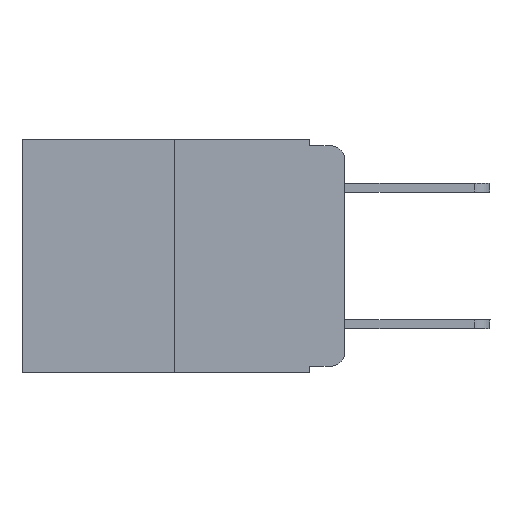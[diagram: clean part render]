
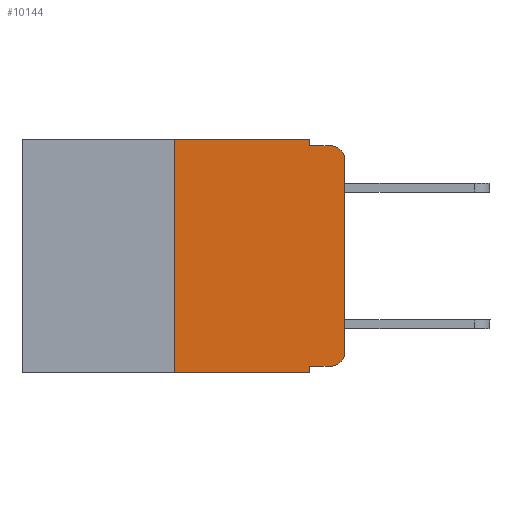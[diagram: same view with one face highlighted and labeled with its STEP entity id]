
A CAD part, left-side view. The second image highlights one B-rep face of the part: STEP entity #10144.
In plain terms, the highlighted planar face has unit normal (-1, 0, 0).
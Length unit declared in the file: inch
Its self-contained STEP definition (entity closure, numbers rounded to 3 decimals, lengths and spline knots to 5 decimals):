
#7 = VERTEX_POINT ( 'NONE', #2720 ) ;
#46 = VERTEX_POINT ( 'NONE', #10222 ) ;
#53 = CARTESIAN_POINT ( 'NONE',  ( 0., 0.473, 0. ) ) ;
#612 = EDGE_CURVE ( 'NONE', #9801, #11192, #1618, .T. ) ;
#665 = FACE_OUTER_BOUND ( 'NONE', #2804, .T. ) ;
#757 = VECTOR ( 'NONE', #13112, 39.37008 ) ;
#1038 = LINE ( 'NONE', #6420, #1865 ) ;
#1233 = AXIS2_PLACEMENT_3D ( 'NONE', #4231, #5417, #5269 ) ;
#1427 = ORIENTED_EDGE ( 'NONE', *, *, #6035, .F. ) ;
#1511 = DIRECTION ( 'NONE',  ( 0., 0., 1. ) ) ;
#1618 = LINE ( 'NONE', #6082, #13371 ) ;
#1855 = CIRCLE ( 'NONE', #6973, 0.02 ) ;
#1865 = VECTOR ( 'NONE', #6332, 39.37008 ) ;
#1982 = CARTESIAN_POINT ( 'NONE',  ( 0., 0.473, 0. ) ) ;
#2523 = ORIENTED_EDGE ( 'NONE', *, *, #2851, .F. ) ;
#2578 = EDGE_CURVE ( 'NONE', #7189, #3994, #7212, .T. ) ;
#2700 = LINE ( 'NONE', #53, #11826 ) ;
#2720 = CARTESIAN_POINT ( 'NONE',  ( 0., 0., -0.313 ) ) ;
#2748 = DIRECTION ( 'NONE',  ( -1., 0., 0. ) ) ;
#2804 = EDGE_LOOP ( 'NONE', ( #5106, #3566, #2523, #9896, #1427, #4032, #12704, #13090, #8368, #5685 ) ) ;
#2851 = EDGE_CURVE ( 'NONE', #3994, #3836, #1038, .T. ) ;
#2891 = DIRECTION ( 'NONE',  ( 0., -1., 0. ) ) ;
#3566 = ORIENTED_EDGE ( 'NONE', *, *, #7395, .T. ) ;
#3836 = VERTEX_POINT ( 'NONE', #6130 ) ;
#3950 = CARTESIAN_POINT ( 'NONE',  ( 0., 0., -0.03 ) ) ;
#3974 = LINE ( 'NONE', #6555, #12480 ) ;
#3994 = VERTEX_POINT ( 'NONE', #9309 ) ;
#4032 = ORIENTED_EDGE ( 'NONE', *, *, #4300, .F. ) ;
#4059 = VERTEX_POINT ( 'NONE', #10612 ) ;
#4231 = CARTESIAN_POINT ( 'NONE',  ( 0., 0.02, -0.03 ) ) ;
#4300 = EDGE_CURVE ( 'NONE', #9801, #4059, #6152, .T. ) ;
#4401 = LINE ( 'NONE', #9603, #6031 ) ;
#4866 = CARTESIAN_POINT ( 'NONE',  ( 0., 0.051, 0. ) ) ;
#4930 = CARTESIAN_POINT ( 'NONE',  ( 0., 0.051, 0. ) ) ;
#4997 = DIRECTION ( 'NONE',  ( 0., 0., -1. ) ) ;
#5106 = ORIENTED_EDGE ( 'NONE', *, *, #6881, .T. ) ;
#5136 = DIRECTION ( 'NONE',  ( 0., -1., 0. ) ) ;
#5169 = AXIS2_PLACEMENT_3D ( 'NONE', #1982, #8321, #12418 ) ;
#5269 = DIRECTION ( 'NONE',  ( 0., 0., -1. ) ) ;
#5340 = DIRECTION ( 'NONE',  ( 0., -1., 0. ) ) ;
#5417 = DIRECTION ( 'NONE',  ( -1., 0., 0. ) ) ;
#5685 = ORIENTED_EDGE ( 'NONE', *, *, #7105, .T. ) ;
#5734 = EDGE_CURVE ( 'NONE', #6526, #11192, #12501, .T. ) ;
#6031 = VECTOR ( 'NONE', #5340, 39.37008 ) ;
#6035 = EDGE_CURVE ( 'NONE', #4059, #7189, #2700, .T. ) ;
#6082 = CARTESIAN_POINT ( 'NONE',  ( 0., 0.473, -0.343 ) ) ;
#6130 = CARTESIAN_POINT ( 'NONE',  ( 0., 0.02, -0.01 ) ) ;
#6152 = LINE ( 'NONE', #9961, #9243 ) ;
#6332 = DIRECTION ( 'NONE',  ( 0., -1., 0. ) ) ;
#6420 = CARTESIAN_POINT ( 'NONE',  ( 0., 0.051, -0.01 ) ) ;
#6502 = DIRECTION ( 'NONE',  ( 0., 0., 1. ) ) ;
#6526 = VERTEX_POINT ( 'NONE', #8882 ) ;
#6555 = CARTESIAN_POINT ( 'NONE',  ( 0., 0., 0. ) ) ;
#6557 = VECTOR ( 'NONE', #4997, 39.37008 ) ;
#6881 = EDGE_CURVE ( 'NONE', #7, #13256, #3974, .T. ) ;
#6973 = AXIS2_PLACEMENT_3D ( 'NONE', #12190, #2748, #13170 ) ;
#7105 = EDGE_CURVE ( 'NONE', #46, #7, #1855, .T. ) ;
#7189 = VERTEX_POINT ( 'NONE', #4930 ) ;
#7212 = LINE ( 'NONE', #4866, #6557 ) ;
#7395 = EDGE_CURVE ( 'NONE', #13256, #3836, #12787, .T. ) ;
#8321 = DIRECTION ( 'NONE',  ( 1., 0., 0. ) ) ;
#8368 = ORIENTED_EDGE ( 'NONE', *, *, #9671, .T. ) ;
#8882 = CARTESIAN_POINT ( 'NONE',  ( 0., 0.051, -0.333 ) ) ;
#9243 = VECTOR ( 'NONE', #1511, 39.37008 ) ;
#9309 = CARTESIAN_POINT ( 'NONE',  ( 0., 0.051, -0.01 ) ) ;
#9603 = CARTESIAN_POINT ( 'NONE',  ( 0., 0.051, -0.333 ) ) ;
#9671 = EDGE_CURVE ( 'NONE', #6526, #46, #4401, .T. ) ;
#9791 = CARTESIAN_POINT ( 'NONE',  ( 0., 0.25, -0.343 ) ) ;
#9801 = VERTEX_POINT ( 'NONE', #9791 ) ;
#9896 = ORIENTED_EDGE ( 'NONE', *, *, #2578, .F. ) ;
#9961 = CARTESIAN_POINT ( 'NONE',  ( 0., 0.25, 0. ) ) ;
#10144 = ADVANCED_FACE ( 'NONE', ( #665 ), #10202, .F. ) ;
#10202 = PLANE ( 'NONE',  #5169 ) ;
#10222 = CARTESIAN_POINT ( 'NONE',  ( 0., 0.02, -0.333 ) ) ;
#10612 = CARTESIAN_POINT ( 'NONE',  ( 0., 0.25, 0. ) ) ;
#10990 = CARTESIAN_POINT ( 'NONE',  ( 0., 0.051, 0. ) ) ;
#11192 = VERTEX_POINT ( 'NONE', #11285 ) ;
#11285 = CARTESIAN_POINT ( 'NONE',  ( 0., 0.051, -0.343 ) ) ;
#11826 = VECTOR ( 'NONE', #5136, 39.37008 ) ;
#12190 = CARTESIAN_POINT ( 'NONE',  ( 0., 0.02, -0.313 ) ) ;
#12418 = DIRECTION ( 'NONE',  ( 0., 0., -1. ) ) ;
#12480 = VECTOR ( 'NONE', #6502, 39.37008 ) ;
#12501 = LINE ( 'NONE', #10990, #757 ) ;
#12704 = ORIENTED_EDGE ( 'NONE', *, *, #612, .T. ) ;
#12787 = CIRCLE ( 'NONE', #1233, 0.02 ) ;
#13090 = ORIENTED_EDGE ( 'NONE', *, *, #5734, .F. ) ;
#13112 = DIRECTION ( 'NONE',  ( 0., 0., -1. ) ) ;
#13170 = DIRECTION ( 'NONE',  ( 0., 0., -1. ) ) ;
#13256 = VERTEX_POINT ( 'NONE', #3950 ) ;
#13371 = VECTOR ( 'NONE', #2891, 39.37008 ) ;
